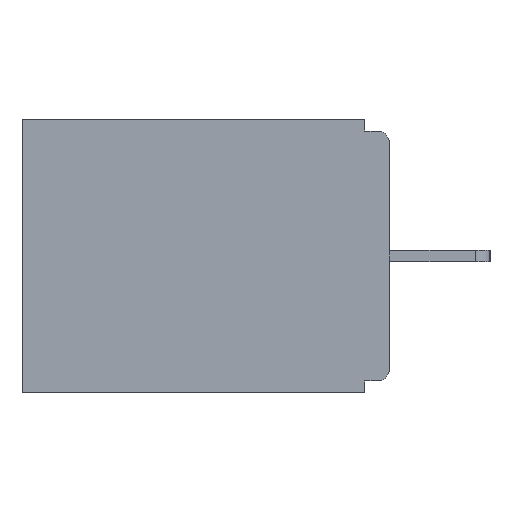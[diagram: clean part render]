
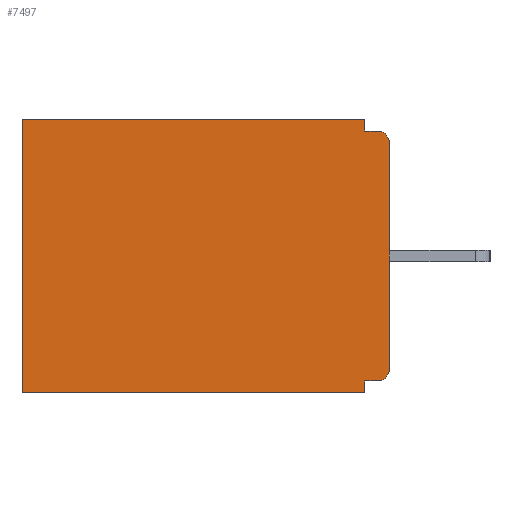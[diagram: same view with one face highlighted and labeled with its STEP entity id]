
A CAD part, left-side view. The second image highlights one B-rep face of the part: STEP entity #7497.
In plain terms, the highlighted planar face has unit normal (-1, 0, 0).
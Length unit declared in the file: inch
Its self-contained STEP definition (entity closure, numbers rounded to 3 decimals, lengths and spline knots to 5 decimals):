
#81 = VERTEX_POINT ( 'NONE', #9486 ) ;
#116 = DIRECTION ( 'NONE',  ( -1., 0., 0. ) ) ;
#468 = EDGE_CURVE ( 'NONE', #8705, #10153, #8370, .T. ) ;
#563 = VERTEX_POINT ( 'NONE', #8141 ) ;
#748 = ORIENTED_EDGE ( 'NONE', *, *, #8792, .F. ) ;
#831 = CARTESIAN_POINT ( 'NONE',  ( 0.298, 0., 0. ) ) ;
#882 = ORIENTED_EDGE ( 'NONE', *, *, #10997, .F. ) ;
#943 = LINE ( 'NONE', #4140, #11456 ) ;
#1048 = DIRECTION ( 'NONE',  ( 0., 0., -1. ) ) ;
#1284 = VERTEX_POINT ( 'NONE', #7534 ) ;
#1771 = DIRECTION ( 'NONE',  ( 0., 1., 0. ) ) ;
#1892 = CARTESIAN_POINT ( 'NONE',  ( 0.298, 0.015, -0.328 ) ) ;
#1999 = CARTESIAN_POINT ( 'NONE',  ( 0.298, 0., -0.343 ) ) ;
#2049 = AXIS2_PLACEMENT_3D ( 'NONE', #7465, #116, #8731 ) ;
#2216 = DIRECTION ( 'NONE',  ( 0., 1., 0. ) ) ;
#2317 = CARTESIAN_POINT ( 'NONE',  ( 0.298, 0., -0.328 ) ) ;
#2366 = EDGE_CURVE ( 'NONE', #3290, #10153, #9856, .T. ) ;
#2467 = VERTEX_POINT ( 'NONE', #5476 ) ;
#2524 = LINE ( 'NONE', #1999, #11638 ) ;
#2550 = CARTESIAN_POINT ( 'NONE',  ( 0.298, 0., 0. ) ) ;
#2592 = CARTESIAN_POINT ( 'NONE',  ( 0.298, 0.031, -0.343 ) ) ;
#2715 = LINE ( 'NONE', #2897, #10514 ) ;
#2897 = CARTESIAN_POINT ( 'NONE',  ( 0.298, 0.031, -0.343 ) ) ;
#3180 = CARTESIAN_POINT ( 'NONE',  ( 0.298, 0.031, -0.015 ) ) ;
#3290 = VERTEX_POINT ( 'NONE', #12316 ) ;
#3392 = ORIENTED_EDGE ( 'NONE', *, *, #2366, .F. ) ;
#4067 = DIRECTION ( 'NONE',  ( 0., -1., 0. ) ) ;
#4140 = CARTESIAN_POINT ( 'NONE',  ( 0.298, 0., -0.015 ) ) ;
#4148 = ORIENTED_EDGE ( 'NONE', *, *, #7714, .F. ) ;
#4463 = LINE ( 'NONE', #8791, #9601 ) ;
#4490 = ORIENTED_EDGE ( 'NONE', *, *, #468, .T. ) ;
#4604 = ORIENTED_EDGE ( 'NONE', *, *, #6560, .F. ) ;
#4623 = ORIENTED_EDGE ( 'NONE', *, *, #7780, .F. ) ;
#4776 = ORIENTED_EDGE ( 'NONE', *, *, #11943, .T. ) ;
#4971 = VECTOR ( 'NONE', #2216, 39.37008 ) ;
#5020 = DIRECTION ( 'NONE',  ( 0., 0., -1. ) ) ;
#5476 = CARTESIAN_POINT ( 'NONE',  ( 0.298, 0.031, 0. ) ) ;
#5572 = ORIENTED_EDGE ( 'NONE', *, *, #8776, .T. ) ;
#5661 = DIRECTION ( 'NONE',  ( 1., 0., 0. ) ) ;
#6078 = PLANE ( 'NONE',  #7587 ) ;
#6560 = EDGE_CURVE ( 'NONE', #563, #7477, #4463, .T. ) ;
#6652 = CARTESIAN_POINT ( 'NONE',  ( 0.298, 0.46, -0.343 ) ) ;
#6793 = VECTOR ( 'NONE', #8620, 39.37008 ) ;
#6870 = VECTOR ( 'NONE', #1771, 39.37008 ) ;
#7414 = DIRECTION ( 'NONE',  ( 0., 1., 0. ) ) ;
#7465 = CARTESIAN_POINT ( 'NONE',  ( 0.298, 0.015, -0.313 ) ) ;
#7477 = VERTEX_POINT ( 'NONE', #2592 ) ;
#7480 = DIRECTION ( 'NONE',  ( 0., 0., -1. ) ) ;
#7497 = ADVANCED_FACE ( 'NONE', ( #10782 ), #6078, .F. ) ;
#7534 = CARTESIAN_POINT ( 'NONE',  ( 0.298, 0.015, -0.015 ) ) ;
#7587 = AXIS2_PLACEMENT_3D ( 'NONE', #2550, #5661, #5020 ) ;
#7714 = EDGE_CURVE ( 'NONE', #8705, #563, #7755, .T. ) ;
#7755 = LINE ( 'NONE', #2317, #4971 ) ;
#7780 = EDGE_CURVE ( 'NONE', #7477, #10572, #2524, .T. ) ;
#8141 = CARTESIAN_POINT ( 'NONE',  ( 0.298, 0.031, -0.328 ) ) ;
#8370 = CIRCLE ( 'NONE', #2049, 0.015 ) ;
#8434 = ORIENTED_EDGE ( 'NONE', *, *, #10389, .T. ) ;
#8597 = EDGE_LOOP ( 'NONE', ( #8434, #748, #882, #5572, #4776, #4623, #4604, #4148, #4490, #3392 ) ) ;
#8620 = DIRECTION ( 'NONE',  ( 0., 0., -1. ) ) ;
#8638 = CARTESIAN_POINT ( 'NONE',  ( 0.298, 0.46, 0. ) ) ;
#8705 = VERTEX_POINT ( 'NONE', #1892 ) ;
#8731 = DIRECTION ( 'NONE',  ( 0., 0., -1. ) ) ;
#8776 = EDGE_CURVE ( 'NONE', #2467, #81, #12063, .T. ) ;
#8791 = CARTESIAN_POINT ( 'NONE',  ( 0.298, 0.031, -0.343 ) ) ;
#8792 = EDGE_CURVE ( 'NONE', #12750, #1284, #943, .T. ) ;
#9485 = CIRCLE ( 'NONE', #12368, 0.015 ) ;
#9486 = CARTESIAN_POINT ( 'NONE',  ( 0.298, 0.46, 0. ) ) ;
#9601 = VECTOR ( 'NONE', #11514, 39.37008 ) ;
#9856 = LINE ( 'NONE', #10193, #12068 ) ;
#10153 = VERTEX_POINT ( 'NONE', #13069 ) ;
#10193 = CARTESIAN_POINT ( 'NONE',  ( 0.298, 0., 0. ) ) ;
#10389 = EDGE_CURVE ( 'NONE', #3290, #1284, #9485, .T. ) ;
#10514 = VECTOR ( 'NONE', #7480, 39.37008 ) ;
#10572 = VERTEX_POINT ( 'NONE', #6652 ) ;
#10782 = FACE_OUTER_BOUND ( 'NONE', #8597, .T. ) ;
#10997 = EDGE_CURVE ( 'NONE', #2467, #12750, #2715, .T. ) ;
#11106 = DIRECTION ( 'NONE',  ( 0., 0., -1. ) ) ;
#11118 = DIRECTION ( 'NONE',  ( -1., 0., 0. ) ) ;
#11120 = CARTESIAN_POINT ( 'NONE',  ( 0.298, 0.015, -0.03 ) ) ;
#11456 = VECTOR ( 'NONE', #4067, 39.37008 ) ;
#11514 = DIRECTION ( 'NONE',  ( 0., 0., -1. ) ) ;
#11638 = VECTOR ( 'NONE', #7414, 39.37008 ) ;
#11943 = EDGE_CURVE ( 'NONE', #81, #10572, #12588, .T. ) ;
#12063 = LINE ( 'NONE', #831, #6870 ) ;
#12068 = VECTOR ( 'NONE', #1048, 39.37008 ) ;
#12316 = CARTESIAN_POINT ( 'NONE',  ( 0.298, 0., -0.03 ) ) ;
#12368 = AXIS2_PLACEMENT_3D ( 'NONE', #11120, #11118, #11106 ) ;
#12588 = LINE ( 'NONE', #8638, #6793 ) ;
#12750 = VERTEX_POINT ( 'NONE', #3180 ) ;
#13069 = CARTESIAN_POINT ( 'NONE',  ( 0.298, 0., -0.313 ) ) ;
